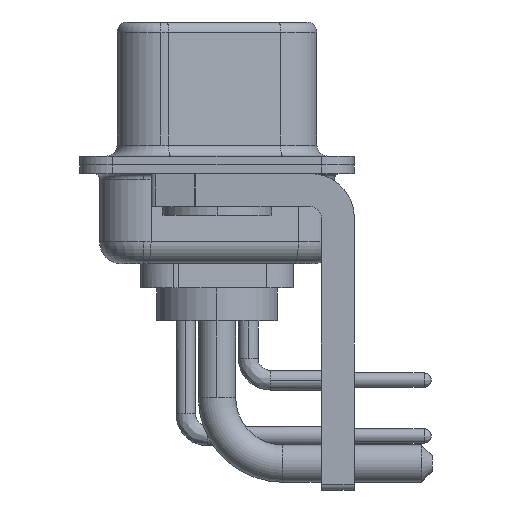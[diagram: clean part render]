
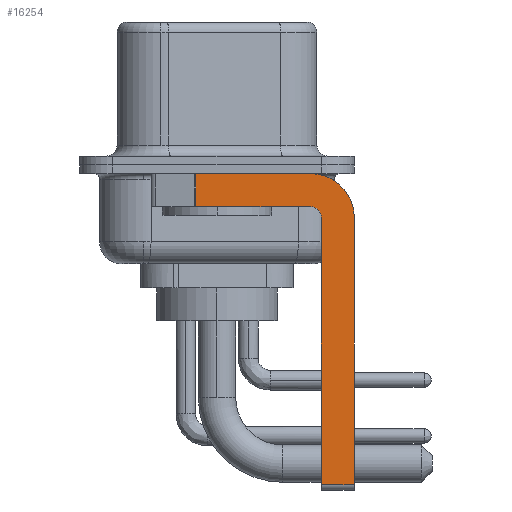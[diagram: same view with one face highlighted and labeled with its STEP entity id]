
A CAD part, left-side view. The second image highlights one B-rep face of the part: STEP entity #16254.
In plain terms, the highlighted planar face has unit normal (-1, 0, 0).
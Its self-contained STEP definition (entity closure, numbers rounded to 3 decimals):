
#49 = LINE ( 'NONE', #8542, #15899 ) ;
#457 = EDGE_CURVE ( 'NONE', #3855, #10348, #49, .T. ) ;
#849 = CARTESIAN_POINT ( 'NONE',  ( -2.9, 0.978, -0.4 ) ) ;
#867 = CARTESIAN_POINT ( 'NONE',  ( -2.9, 0.978, -1.9 ) ) ;
#1308 = CARTESIAN_POINT ( 'NONE',  ( -2.9, -4.75, -14.55 ) ) ;
#1591 = DIRECTION ( 'NONE',  ( 0., 0., 1. ) ) ;
#1831 = CARTESIAN_POINT ( 'NONE',  ( -2.9, -4.25, -1.9 ) ) ;
#2665 = DIRECTION ( 'NONE',  ( 0., -1., 0. ) ) ;
#2820 = DIRECTION ( 'NONE',  ( 0., 0., -1. ) ) ;
#2983 = CARTESIAN_POINT ( 'NONE',  ( -2.9, -4.75, -2.4 ) ) ;
#3107 = EDGE_CURVE ( 'NONE', #10837, #3855, #16922, .T. ) ;
#3251 = DIRECTION ( 'NONE',  ( 0., -1., 0. ) ) ;
#3409 = CARTESIAN_POINT ( 'NONE',  ( -2.9, -4.75, -14.8 ) ) ;
#3618 = AXIS2_PLACEMENT_3D ( 'NONE', #23037, #25004, #5917 ) ;
#3801 = EDGE_LOOP ( 'NONE', ( #12353, #6506, #16326, #7607, #6534, #14092, #9286, #4956 ) ) ;
#3855 = VERTEX_POINT ( 'NONE', #1831 ) ;
#4159 = DIRECTION ( 'NONE',  ( 0., 0., -1. ) ) ;
#4378 = DIRECTION ( 'NONE',  ( 0., 0., 1. ) ) ;
#4643 = LINE ( 'NONE', #7003, #15728 ) ;
#4956 = ORIENTED_EDGE ( 'NONE', *, *, #21206, .F. ) ;
#5642 = LINE ( 'NONE', #3409, #6863 ) ;
#5850 = VERTEX_POINT ( 'NONE', #10138 ) ;
#5917 = DIRECTION ( 'NONE',  ( 0., 0., -1. ) ) ;
#6468 = DIRECTION ( 'NONE',  ( -1., 0., 0. ) ) ;
#6506 = ORIENTED_EDGE ( 'NONE', *, *, #16499, .T. ) ;
#6534 = ORIENTED_EDGE ( 'NONE', *, *, #18992, .F. ) ;
#6863 = VECTOR ( 'NONE', #1591, 1000. ) ;
#7003 = CARTESIAN_POINT ( 'NONE',  ( -2.9, -4.25, -14.55 ) ) ;
#7607 = ORIENTED_EDGE ( 'NONE', *, *, #3107, .F. ) ;
#8025 = DIRECTION ( 'NONE',  ( 0., 0., -1. ) ) ;
#8539 = AXIS2_PLACEMENT_3D ( 'NONE', #9704, #18478, #8025 ) ;
#8542 = CARTESIAN_POINT ( 'NONE',  ( -2.9, -4.25, -1.9 ) ) ;
#8557 = CARTESIAN_POINT ( 'NONE',  ( -2.9, -4.25, -2.4 ) ) ;
#9286 = ORIENTED_EDGE ( 'NONE', *, *, #18162, .F. ) ;
#9704 = CARTESIAN_POINT ( 'NONE',  ( -2.9, -4.25, -2.4 ) ) ;
#10009 = VERTEX_POINT ( 'NONE', #24517 ) ;
#10138 = CARTESIAN_POINT ( 'NONE',  ( -2.9, -4.25, -0.4 ) ) ;
#10287 = LINE ( 'NONE', #16434, #21513 ) ;
#10348 = VERTEX_POINT ( 'NONE', #19614 ) ;
#10837 = VERTEX_POINT ( 'NONE', #2983 ) ;
#12019 = AXIS2_PLACEMENT_3D ( 'NONE', #8557, #6468, #4378 ) ;
#12353 = ORIENTED_EDGE ( 'NONE', *, *, #20321, .F. ) ;
#12930 = VERTEX_POINT ( 'NONE', #1308 ) ;
#13904 = VECTOR ( 'NONE', #2820, 1000. ) ;
#14092 = ORIENTED_EDGE ( 'NONE', *, *, #17459, .T. ) ;
#15728 = VECTOR ( 'NONE', #2665, 1000. ) ;
#15899 = VECTOR ( 'NONE', #17063, 1000. ) ;
#16254 = ADVANCED_FACE ( 'NONE', ( #20697 ), #19001, .F. ) ;
#16326 = ORIENTED_EDGE ( 'NONE', *, *, #457, .F. ) ;
#16434 = CARTESIAN_POINT ( 'NONE',  ( -2.9, -6.25, -2.4 ) ) ;
#16499 = EDGE_CURVE ( 'NONE', #20610, #10348, #18021, .T. ) ;
#16922 = CIRCLE ( 'NONE', #12019, 0.5 ) ;
#17063 = DIRECTION ( 'NONE',  ( 0., 1., 0. ) ) ;
#17459 = EDGE_CURVE ( 'NONE', #12930, #24211, #4643, .T. ) ;
#18021 = LINE ( 'NONE', #867, #13904 ) ;
#18162 = EDGE_CURVE ( 'NONE', #10009, #24211, #10287, .T. ) ;
#18478 = DIRECTION ( 'NONE',  ( 1., 0., 0. ) ) ;
#18992 = EDGE_CURVE ( 'NONE', #12930, #10837, #5642, .T. ) ;
#19001 = PLANE ( 'NONE',  #3618 ) ;
#19614 = CARTESIAN_POINT ( 'NONE',  ( -2.9, 0.978, -1.9 ) ) ;
#20321 = EDGE_CURVE ( 'NONE', #20610, #5850, #22752, .T. ) ;
#20401 = CARTESIAN_POINT ( 'NONE',  ( -2.9, 3., -0.4 ) ) ;
#20580 = CIRCLE ( 'NONE', #8539, 2. ) ;
#20610 = VERTEX_POINT ( 'NONE', #849 ) ;
#20697 = FACE_OUTER_BOUND ( 'NONE', #3801, .T. ) ;
#21206 = EDGE_CURVE ( 'NONE', #5850, #10009, #20580, .T. ) ;
#21513 = VECTOR ( 'NONE', #4159, 1000. ) ;
#22752 = LINE ( 'NONE', #20401, #24089 ) ;
#22957 = CARTESIAN_POINT ( 'NONE',  ( -2.9, -6.25, -14.55 ) ) ;
#23037 = CARTESIAN_POINT ( 'NONE',  ( -2.9, -4.25, -2.4 ) ) ;
#24089 = VECTOR ( 'NONE', #3251, 1000. ) ;
#24211 = VERTEX_POINT ( 'NONE', #22957 ) ;
#24517 = CARTESIAN_POINT ( 'NONE',  ( -2.9, -6.25, -2.4 ) ) ;
#25004 = DIRECTION ( 'NONE',  ( 1., 0., 0. ) ) ;
